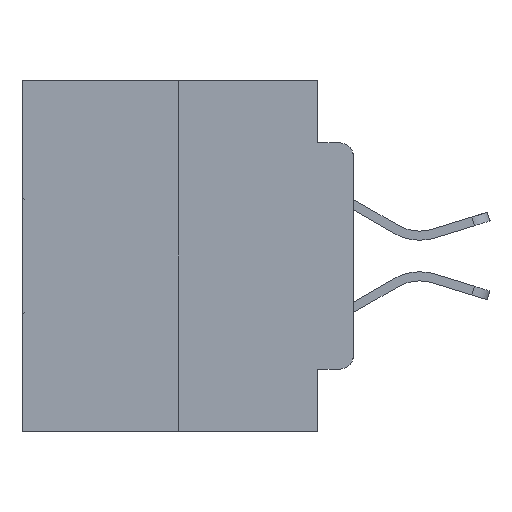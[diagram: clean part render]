
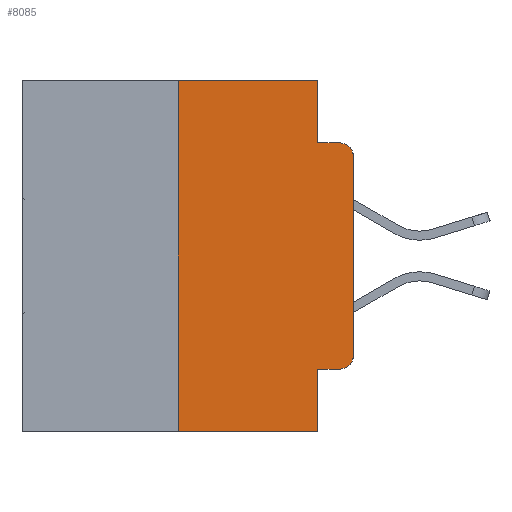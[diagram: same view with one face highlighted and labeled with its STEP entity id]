
A CAD part, left-side view. The second image highlights one B-rep face of the part: STEP entity #8085.
In plain terms, the highlighted planar face has unit normal (-1, 0, 0).
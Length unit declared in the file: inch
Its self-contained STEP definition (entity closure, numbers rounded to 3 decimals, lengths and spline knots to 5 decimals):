
#372 = ORIENTED_EDGE ( 'NONE', *, *, #18010, .F. ) ;
#536 = AXIS2_PLACEMENT_3D ( 'NONE', #20061, #17644, #22329 ) ;
#723 = CARTESIAN_POINT ( 'NONE',  ( 0., 0.051, -0.0885 ) ) ;
#913 = LINE ( 'NONE', #23250, #29466 ) ;
#1070 = CARTESIAN_POINT ( 'NONE',  ( 0., 0.25, -0.5 ) ) ;
#2407 = ORIENTED_EDGE ( 'NONE', *, *, #29360, .F. ) ;
#2669 = VECTOR ( 'NONE', #13711, 39.37008 ) ;
#2797 = DIRECTION ( 'NONE',  ( 0., -1., 0. ) ) ;
#4502 = VECTOR ( 'NONE', #2797, 39.37008 ) ;
#4575 = CARTESIAN_POINT ( 'NONE',  ( 0., 0., -0.1085 ) ) ;
#5286 = CARTESIAN_POINT ( 'NONE',  ( 0., 0.25, 0. ) ) ;
#5410 = LINE ( 'NONE', #17147, #17163 ) ;
#5561 = DIRECTION ( 'NONE',  ( 0., 0., 1. ) ) ;
#5996 = CARTESIAN_POINT ( 'NONE',  ( 0., 0.051, 0. ) ) ;
#6154 = LINE ( 'NONE', #5996, #2669 ) ;
#6876 = ORIENTED_EDGE ( 'NONE', *, *, #24273, .T. ) ;
#7074 = ORIENTED_EDGE ( 'NONE', *, *, #13189, .T. ) ;
#7485 = VECTOR ( 'NONE', #8148, 39.37008 ) ;
#8085 = ADVANCED_FACE ( 'NONE', ( #22638 ), #22022, .F. ) ;
#8148 = DIRECTION ( 'NONE',  ( 0., -1., 0. ) ) ;
#8533 = EDGE_CURVE ( 'NONE', #12080, #11555, #10059, .T. ) ;
#9319 = ORIENTED_EDGE ( 'NONE', *, *, #24201, .F. ) ;
#9541 = LINE ( 'NONE', #19331, #26968 ) ;
#9833 = DIRECTION ( 'NONE',  ( 0., 0., -1. ) ) ;
#9870 = CARTESIAN_POINT ( 'NONE',  ( 0., 0.051, 0. ) ) ;
#10059 = LINE ( 'NONE', #10226, #11279 ) ;
#10216 = VECTOR ( 'NONE', #5561, 39.37008 ) ;
#10226 = CARTESIAN_POINT ( 'NONE',  ( 0., 0.051, -0.4115 ) ) ;
#11279 = VECTOR ( 'NONE', #29850, 39.37008 ) ;
#11555 = VERTEX_POINT ( 'NONE', #26031 ) ;
#11675 = DIRECTION ( 'NONE',  ( -1., 0., 0. ) ) ;
#12080 = VERTEX_POINT ( 'NONE', #19465 ) ;
#12646 = VERTEX_POINT ( 'NONE', #1070 ) ;
#13022 = CIRCLE ( 'NONE', #31043, 0.02 ) ;
#13189 = EDGE_CURVE ( 'NONE', #19059, #20946, #23209, .T. ) ;
#13711 = DIRECTION ( 'NONE',  ( 0., 0., -1. ) ) ;
#13771 = CARTESIAN_POINT ( 'NONE',  ( 0., 0.02, -0.3915 ) ) ;
#14436 = EDGE_CURVE ( 'NONE', #16130, #20946, #24859, .T. ) ;
#15218 = LINE ( 'NONE', #27619, #7485 ) ;
#15418 = ORIENTED_EDGE ( 'NONE', *, *, #8533, .T. ) ;
#15493 = CARTESIAN_POINT ( 'NONE',  ( 0., 0.02, -0.1085 ) ) ;
#15771 = EDGE_CURVE ( 'NONE', #21981, #19059, #19396, .T. ) ;
#16130 = VERTEX_POINT ( 'NONE', #27430 ) ;
#17147 = CARTESIAN_POINT ( 'NONE',  ( 0., 0.473, -0.5 ) ) ;
#17163 = VECTOR ( 'NONE', #26982, 39.37008 ) ;
#17644 = DIRECTION ( 'NONE',  ( 1., 0., 0. ) ) ;
#18010 = EDGE_CURVE ( 'NONE', #12080, #21022, #6154, .T. ) ;
#18051 = DIRECTION ( 'NONE',  ( 0., 0., -1. ) ) ;
#19059 = VERTEX_POINT ( 'NONE', #4575 ) ;
#19331 = CARTESIAN_POINT ( 'NONE',  ( 0., 0.051, 0. ) ) ;
#19396 = LINE ( 'NONE', #29235, #10216 ) ;
#19465 = CARTESIAN_POINT ( 'NONE',  ( 0., 0.051, -0.4115 ) ) ;
#20061 = CARTESIAN_POINT ( 'NONE',  ( 0., 0.473, 0. ) ) ;
#20946 = VERTEX_POINT ( 'NONE', #24432 ) ;
#21022 = VERTEX_POINT ( 'NONE', #28120 ) ;
#21981 = VERTEX_POINT ( 'NONE', #23651 ) ;
#22022 = PLANE ( 'NONE',  #536 ) ;
#22117 = VERTEX_POINT ( 'NONE', #5286 ) ;
#22272 = EDGE_LOOP ( 'NONE', ( #31428, #7074, #23664, #2407, #27849, #9319, #29480, #372, #15418, #6876 ) ) ;
#22329 = DIRECTION ( 'NONE',  ( 0., 0., -1. ) ) ;
#22638 = FACE_OUTER_BOUND ( 'NONE', #22272, .T. ) ;
#22905 = DIRECTION ( 'NONE',  ( -1., 0., 0. ) ) ;
#23209 = CIRCLE ( 'NONE', #25790, 0.02 ) ;
#23250 = CARTESIAN_POINT ( 'NONE',  ( 0., 0.25, 0. ) ) ;
#23420 = DIRECTION ( 'NONE',  ( 0., 0., -1. ) ) ;
#23651 = CARTESIAN_POINT ( 'NONE',  ( 0., 0., -0.3915 ) ) ;
#23664 = ORIENTED_EDGE ( 'NONE', *, *, #14436, .F. ) ;
#24201 = EDGE_CURVE ( 'NONE', #12646, #22117, #913, .T. ) ;
#24273 = EDGE_CURVE ( 'NONE', #11555, #21981, #13022, .T. ) ;
#24432 = CARTESIAN_POINT ( 'NONE',  ( 0., 0.02, -0.0885 ) ) ;
#24859 = LINE ( 'NONE', #723, #4502 ) ;
#25790 = AXIS2_PLACEMENT_3D ( 'NONE', #15493, #22905, #18051 ) ;
#26031 = CARTESIAN_POINT ( 'NONE',  ( 0., 0.02, -0.4115 ) ) ;
#26968 = VECTOR ( 'NONE', #9833, 39.37008 ) ;
#26982 = DIRECTION ( 'NONE',  ( 0., -1., 0. ) ) ;
#27430 = CARTESIAN_POINT ( 'NONE',  ( 0., 0.051, -0.0885 ) ) ;
#27619 = CARTESIAN_POINT ( 'NONE',  ( 0., 0.473, 0. ) ) ;
#27849 = ORIENTED_EDGE ( 'NONE', *, *, #27932, .F. ) ;
#27932 = EDGE_CURVE ( 'NONE', #22117, #28234, #15218, .T. ) ;
#28092 = DIRECTION ( 'NONE',  ( 0., 0., 1. ) ) ;
#28120 = CARTESIAN_POINT ( 'NONE',  ( 0., 0.051, -0.5 ) ) ;
#28234 = VERTEX_POINT ( 'NONE', #9870 ) ;
#29124 = EDGE_CURVE ( 'NONE', #12646, #21022, #5410, .T. ) ;
#29235 = CARTESIAN_POINT ( 'NONE',  ( 0., 0., 0. ) ) ;
#29360 = EDGE_CURVE ( 'NONE', #28234, #16130, #9541, .T. ) ;
#29466 = VECTOR ( 'NONE', #28092, 39.37008 ) ;
#29480 = ORIENTED_EDGE ( 'NONE', *, *, #29124, .T. ) ;
#29850 = DIRECTION ( 'NONE',  ( 0., -1., 0. ) ) ;
#31043 = AXIS2_PLACEMENT_3D ( 'NONE', #13771, #11675, #23420 ) ;
#31428 = ORIENTED_EDGE ( 'NONE', *, *, #15771, .T. ) ;
